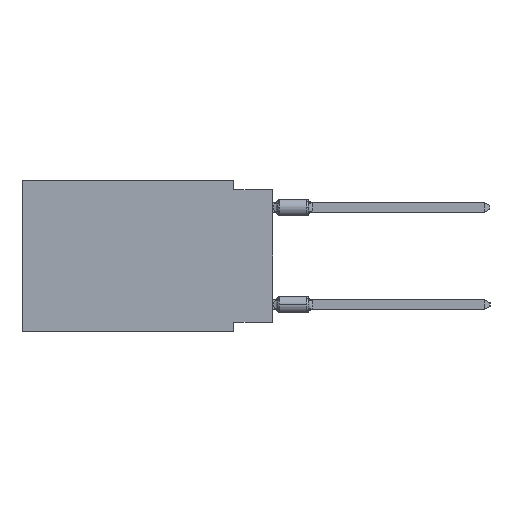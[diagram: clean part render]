
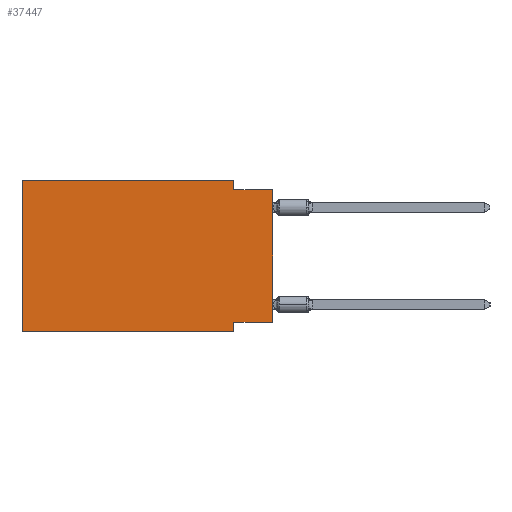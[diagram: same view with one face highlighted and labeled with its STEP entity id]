
A CAD part, left-side view. The second image highlights one B-rep face of the part: STEP entity #37447.
In plain terms, the highlighted planar face has unit normal (-1, 0, 0).
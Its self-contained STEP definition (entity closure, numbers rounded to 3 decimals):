
#47 = VERTEX_POINT ( 'NONE', #24157 ) ;
#558 = VECTOR ( 'NONE', #2770, 1000. ) ;
#1716 = ORIENTED_EDGE ( 'NONE', *, *, #53677, .F. ) ;
#2468 = CARTESIAN_POINT ( 'NONE',  ( 0., 2.54, -9.271 ) ) ;
#2770 = DIRECTION ( 'NONE',  ( 0., -1., 0. ) ) ;
#3141 = VERTEX_POINT ( 'NONE', #54089 ) ;
#6415 = ORIENTED_EDGE ( 'NONE', *, *, #9724, .F. ) ;
#6917 = DIRECTION ( 'NONE',  ( 1., 0., 0. ) ) ;
#7501 = CARTESIAN_POINT ( 'NONE',  ( 0., 2.54, -9.906 ) ) ;
#7532 = LINE ( 'NONE', #16897, #39621 ) ;
#8262 = EDGE_LOOP ( 'NONE', ( #13474, #33581, #27927, #1716, #33792, #37704, #41107, #6415 ) ) ;
#8996 = VERTEX_POINT ( 'NONE', #44138 ) ;
#9392 = VECTOR ( 'NONE', #11320, 1000. ) ;
#9443 = EDGE_CURVE ( 'NONE', #41113, #57354, #7532, .T. ) ;
#9724 = EDGE_CURVE ( 'NONE', #8996, #52496, #33708, .T. ) ;
#11316 = CARTESIAN_POINT ( 'NONE',  ( 0., 16.383, 0. ) ) ;
#11320 = DIRECTION ( 'NONE',  ( 0., 0., -1. ) ) ;
#11953 = EDGE_CURVE ( 'NONE', #12890, #3141, #39290, .T. ) ;
#12890 = VERTEX_POINT ( 'NONE', #21339 ) ;
#13066 = CARTESIAN_POINT ( 'NONE',  ( 0., 16.383, -9.906 ) ) ;
#13474 = ORIENTED_EDGE ( 'NONE', *, *, #22939, .T. ) ;
#13833 = AXIS2_PLACEMENT_3D ( 'NONE', #11316, #6917, #32659 ) ;
#16231 = DIRECTION ( 'NONE',  ( 0., 0., 1. ) ) ;
#16897 = CARTESIAN_POINT ( 'NONE',  ( 0., 0., -0.635 ) ) ;
#17092 = CARTESIAN_POINT ( 'NONE',  ( 0., 16.383, 0. ) ) ;
#17646 = CARTESIAN_POINT ( 'NONE',  ( 0., 0., 0. ) ) ;
#20850 = CARTESIAN_POINT ( 'NONE',  ( 0., 0., -9.271 ) ) ;
#21339 = CARTESIAN_POINT ( 'NONE',  ( 0., 16.383, -9.906 ) ) ;
#22611 = EDGE_CURVE ( 'NONE', #12890, #47, #57787, .T. ) ;
#22939 = EDGE_CURVE ( 'NONE', #8996, #57354, #56818, .T. ) ;
#24157 = CARTESIAN_POINT ( 'NONE',  ( 0., 2.54, -9.906 ) ) ;
#27927 = ORIENTED_EDGE ( 'NONE', *, *, #44673, .F. ) ;
#27963 = EDGE_CURVE ( 'NONE', #52496, #47, #51072, .T. ) ;
#30895 = DIRECTION ( 'NONE',  ( 0., -1., 0. ) ) ;
#32659 = DIRECTION ( 'NONE',  ( 0., 0., -1. ) ) ;
#33581 = ORIENTED_EDGE ( 'NONE', *, *, #9443, .F. ) ;
#33587 = VECTOR ( 'NONE', #47816, 1000. ) ;
#33708 = LINE ( 'NONE', #20850, #45225 ) ;
#33792 = ORIENTED_EDGE ( 'NONE', *, *, #11953, .F. ) ;
#34420 = DIRECTION ( 'NONE',  ( 0., -1., 0. ) ) ;
#37037 = FACE_OUTER_BOUND ( 'NONE', #8262, .T. ) ;
#37447 = ADVANCED_FACE ( 'NONE', ( #37037 ), #54884, .F. ) ;
#37704 = ORIENTED_EDGE ( 'NONE', *, *, #22611, .T. ) ;
#38378 = VECTOR ( 'NONE', #30895, 1000. ) ;
#38381 = DIRECTION ( 'NONE',  ( 0., 1., 0. ) ) ;
#38745 = VECTOR ( 'NONE', #16231, 1000. ) ;
#39030 = CARTESIAN_POINT ( 'NONE',  ( 0., 2.54, -0.635 ) ) ;
#39290 = LINE ( 'NONE', #17092, #38745 ) ;
#39621 = VECTOR ( 'NONE', #34420, 1000. ) ;
#41107 = ORIENTED_EDGE ( 'NONE', *, *, #27963, .F. ) ;
#41113 = VERTEX_POINT ( 'NONE', #39030 ) ;
#42177 = VECTOR ( 'NONE', #47765, 1000. ) ;
#42280 = LINE ( 'NONE', #51626, #33587 ) ;
#42835 = LINE ( 'NONE', #55996, #558 ) ;
#44138 = CARTESIAN_POINT ( 'NONE',  ( 0., 0., -9.271 ) ) ;
#44673 = EDGE_CURVE ( 'NONE', #56932, #41113, #42280, .T. ) ;
#45225 = VECTOR ( 'NONE', #38381, 1000. ) ;
#46935 = CARTESIAN_POINT ( 'NONE',  ( 0., 2.54, 0. ) ) ;
#47765 = DIRECTION ( 'NONE',  ( 0., 0., 1. ) ) ;
#47816 = DIRECTION ( 'NONE',  ( 0., 0., -1. ) ) ;
#49400 = CARTESIAN_POINT ( 'NONE',  ( 0., 0., -0.635 ) ) ;
#51072 = LINE ( 'NONE', #7501, #9392 ) ;
#51626 = CARTESIAN_POINT ( 'NONE',  ( 0., 2.54, 0. ) ) ;
#52496 = VERTEX_POINT ( 'NONE', #2468 ) ;
#53677 = EDGE_CURVE ( 'NONE', #3141, #56932, #42835, .T. ) ;
#54089 = CARTESIAN_POINT ( 'NONE',  ( 0., 16.383, 0. ) ) ;
#54884 = PLANE ( 'NONE',  #13833 ) ;
#55996 = CARTESIAN_POINT ( 'NONE',  ( 0., 16.383, 0. ) ) ;
#56818 = LINE ( 'NONE', #17646, #42177 ) ;
#56932 = VERTEX_POINT ( 'NONE', #46935 ) ;
#57354 = VERTEX_POINT ( 'NONE', #49400 ) ;
#57787 = LINE ( 'NONE', #13066, #38378 ) ;
